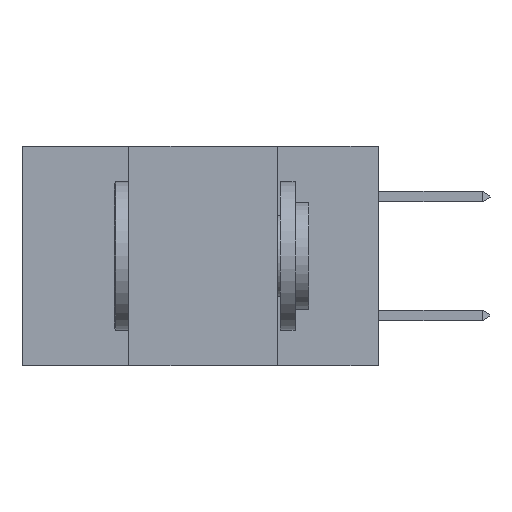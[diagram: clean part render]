
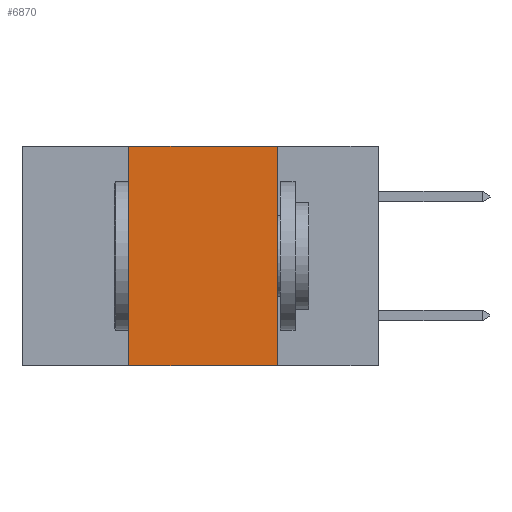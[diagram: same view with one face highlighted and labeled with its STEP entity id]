
A CAD part, left-side view. The second image highlights one B-rep face of the part: STEP entity #6870.
In plain terms, the highlighted planar face has unit normal (-1, 0, 0).
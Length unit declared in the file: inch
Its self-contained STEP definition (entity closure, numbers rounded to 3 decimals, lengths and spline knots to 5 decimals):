
#134 = EDGE_CURVE ( 'NONE', #18054, #18031, #16302, .T. ) ;
#191 = CARTESIAN_POINT ( 'NONE',  ( 0., 0.17, 0. ) ) ;
#662 = LINE ( 'NONE', #191, #16794 ) ;
#1183 = EDGE_CURVE ( 'NONE', #9024, #7109, #662, .T. ) ;
#2773 = CARTESIAN_POINT ( 'NONE',  ( 0., 0.42, -0.37 ) ) ;
#5022 = AXIS2_PLACEMENT_3D ( 'NONE', #8674, #10373, #12269 ) ;
#5202 = EDGE_LOOP ( 'NONE', ( #10456, #18808, #16848, #19435 ) ) ;
#5760 = DIRECTION ( 'NONE',  ( 0., -1., 0. ) ) ;
#6870 = ADVANCED_FACE ( 'NONE', ( #20202 ), #19000, .F. ) ;
#7109 = VERTEX_POINT ( 'NONE', #17889 ) ;
#7379 = EDGE_CURVE ( 'NONE', #18054, #7109, #15952, .T. ) ;
#8674 = CARTESIAN_POINT ( 'NONE',  ( 0., 0.6, 0. ) ) ;
#9024 = VERTEX_POINT ( 'NONE', #12710 ) ;
#10373 = DIRECTION ( 'NONE',  ( 1., 0., 0. ) ) ;
#10456 = ORIENTED_EDGE ( 'NONE', *, *, #1183, .F. ) ;
#10479 = VECTOR ( 'NONE', #5760, 39.37008 ) ;
#10913 = CARTESIAN_POINT ( 'NONE',  ( 0., 0.6, 0. ) ) ;
#11780 = VECTOR ( 'NONE', #18430, 39.37008 ) ;
#12127 = DIRECTION ( 'NONE',  ( 0., 0., -1. ) ) ;
#12269 = DIRECTION ( 'NONE',  ( 0., 0., -1. ) ) ;
#12710 = CARTESIAN_POINT ( 'NONE',  ( 0., 0.17, 0. ) ) ;
#12877 = DIRECTION ( 'NONE',  ( 0., -1., 0. ) ) ;
#14971 = EDGE_CURVE ( 'NONE', #18031, #9024, #19725, .T. ) ;
#15952 = LINE ( 'NONE', #19739, #17259 ) ;
#16302 = LINE ( 'NONE', #20076, #11780 ) ;
#16794 = VECTOR ( 'NONE', #12127, 39.37008 ) ;
#16848 = ORIENTED_EDGE ( 'NONE', *, *, #134, .F. ) ;
#17259 = VECTOR ( 'NONE', #12877, 39.37008 ) ;
#17889 = CARTESIAN_POINT ( 'NONE',  ( 0., 0.17, -0.37 ) ) ;
#18031 = VERTEX_POINT ( 'NONE', #19329 ) ;
#18054 = VERTEX_POINT ( 'NONE', #2773 ) ;
#18430 = DIRECTION ( 'NONE',  ( 0., 0., 1. ) ) ;
#18808 = ORIENTED_EDGE ( 'NONE', *, *, #14971, .F. ) ;
#19000 = PLANE ( 'NONE',  #5022 ) ;
#19329 = CARTESIAN_POINT ( 'NONE',  ( 0., 0.42, 0. ) ) ;
#19435 = ORIENTED_EDGE ( 'NONE', *, *, #7379, .T. ) ;
#19725 = LINE ( 'NONE', #10913, #10479 ) ;
#19739 = CARTESIAN_POINT ( 'NONE',  ( 0., 0.6, -0.37 ) ) ;
#20076 = CARTESIAN_POINT ( 'NONE',  ( 0., 0.42, 0. ) ) ;
#20202 = FACE_OUTER_BOUND ( 'NONE', #5202, .T. ) ;
